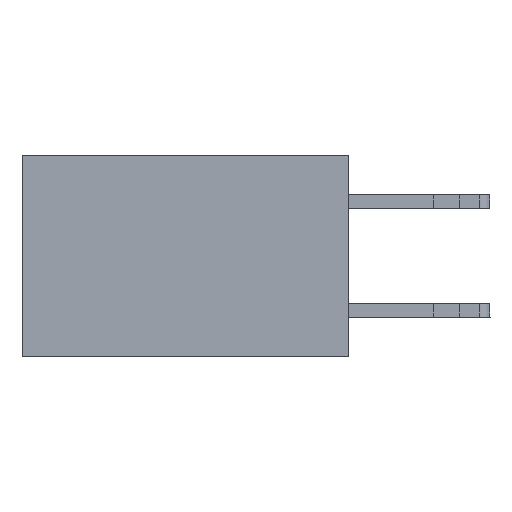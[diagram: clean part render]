
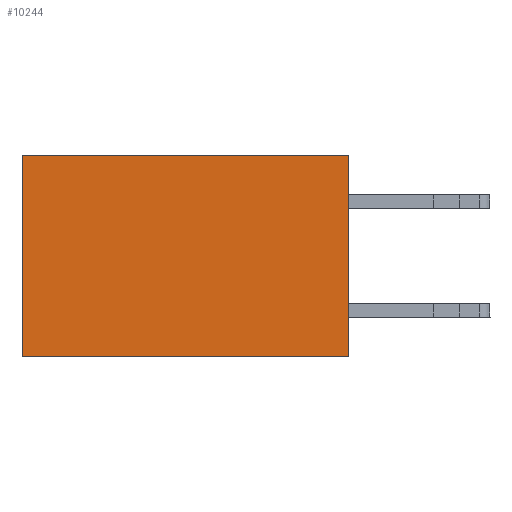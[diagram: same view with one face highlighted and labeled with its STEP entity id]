
A CAD part, left-side view. The second image highlights one B-rep face of the part: STEP entity #10244.
In plain terms, the highlighted planar face has unit normal (-1, 0, 0).
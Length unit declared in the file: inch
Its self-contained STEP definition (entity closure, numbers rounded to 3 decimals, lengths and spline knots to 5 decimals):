
#518 = LINE ( 'NONE', #8954, #13255 ) ;
#1305 = LINE ( 'NONE', #7531, #11432 ) ;
#1512 = VERTEX_POINT ( 'NONE', #4208 ) ;
#2790 = DIRECTION ( 'NONE',  ( 0., 1., 0. ) ) ;
#3133 = EDGE_CURVE ( 'NONE', #1512, #7136, #7480, .T. ) ;
#3313 = VECTOR ( 'NONE', #6678, 39.37008 ) ;
#3599 = CARTESIAN_POINT ( 'NONE',  ( 0.298, 0., 0. ) ) ;
#4208 = CARTESIAN_POINT ( 'NONE',  ( 0.298, 0., -0.37 ) ) ;
#4551 = VECTOR ( 'NONE', #2790, 39.37008 ) ;
#4594 = PLANE ( 'NONE',  #7686 ) ;
#5500 = DIRECTION ( 'NONE',  ( 0., 0., -1. ) ) ;
#5528 = EDGE_LOOP ( 'NONE', ( #12343, #9944, #12188, #7343 ) ) ;
#6508 = CARTESIAN_POINT ( 'NONE',  ( 0.298, 0.6, -0.37 ) ) ;
#6559 = DIRECTION ( 'NONE',  ( 0., 0., -1. ) ) ;
#6678 = DIRECTION ( 'NONE',  ( 0., 1., 0. ) ) ;
#6727 = DIRECTION ( 'NONE',  ( 1., 0., 0. ) ) ;
#6760 = CARTESIAN_POINT ( 'NONE',  ( 0.298, 0., 0. ) ) ;
#6766 = DIRECTION ( 'NONE',  ( 0., 0., -1. ) ) ;
#7031 = CARTESIAN_POINT ( 'NONE',  ( 0.298, 0.6, 0. ) ) ;
#7136 = VERTEX_POINT ( 'NONE', #6508 ) ;
#7343 = ORIENTED_EDGE ( 'NONE', *, *, #10689, .T. ) ;
#7389 = EDGE_CURVE ( 'NONE', #10294, #7136, #518, .T. ) ;
#7480 = LINE ( 'NONE', #10037, #4551 ) ;
#7531 = CARTESIAN_POINT ( 'NONE',  ( 0.298, 0., 0. ) ) ;
#7686 = AXIS2_PLACEMENT_3D ( 'NONE', #3599, #6727, #6559 ) ;
#8549 = FACE_OUTER_BOUND ( 'NONE', #5528, .T. ) ;
#8954 = CARTESIAN_POINT ( 'NONE',  ( 0.298, 0.6, 0. ) ) ;
#9944 = ORIENTED_EDGE ( 'NONE', *, *, #3133, .F. ) ;
#10037 = CARTESIAN_POINT ( 'NONE',  ( 0.298, 0., -0.37 ) ) ;
#10244 = ADVANCED_FACE ( 'NONE', ( #8549 ), #4594, .F. ) ;
#10294 = VERTEX_POINT ( 'NONE', #7031 ) ;
#10537 = EDGE_CURVE ( 'NONE', #10629, #1512, #1305, .T. ) ;
#10629 = VERTEX_POINT ( 'NONE', #12727 ) ;
#10689 = EDGE_CURVE ( 'NONE', #10629, #10294, #12079, .T. ) ;
#11432 = VECTOR ( 'NONE', #5500, 39.37008 ) ;
#12079 = LINE ( 'NONE', #6760, #3313 ) ;
#12188 = ORIENTED_EDGE ( 'NONE', *, *, #10537, .F. ) ;
#12343 = ORIENTED_EDGE ( 'NONE', *, *, #7389, .T. ) ;
#12727 = CARTESIAN_POINT ( 'NONE',  ( 0.298, 0., 0. ) ) ;
#13255 = VECTOR ( 'NONE', #6766, 39.37008 ) ;
